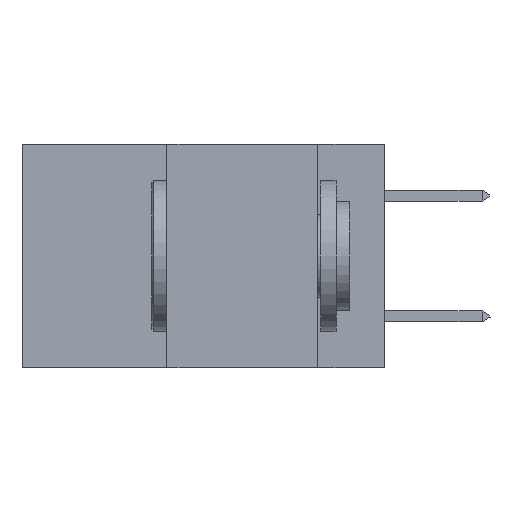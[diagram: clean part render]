
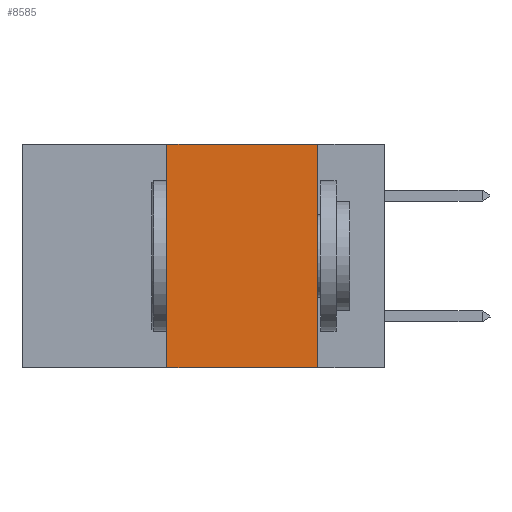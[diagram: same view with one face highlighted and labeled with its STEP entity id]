
A CAD part, left-side view. The second image highlights one B-rep face of the part: STEP entity #8585.
In plain terms, the highlighted planar face has unit normal (-1, 0, 0).
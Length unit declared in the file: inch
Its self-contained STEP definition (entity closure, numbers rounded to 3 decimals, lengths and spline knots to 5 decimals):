
#715 = EDGE_CURVE ( 'NONE', #1308, #7889, #6075, .T. ) ;
#1003 = DIRECTION ( 'NONE',  ( 0., 0., -1. ) ) ;
#1058 = EDGE_CURVE ( 'NONE', #6258, #7382, #5250, .T. ) ;
#1162 = CARTESIAN_POINT ( 'NONE',  ( 0., 0.36, 0. ) ) ;
#1308 = VERTEX_POINT ( 'NONE', #2373 ) ;
#1417 = CARTESIAN_POINT ( 'NONE',  ( 0., 0.6, 0. ) ) ;
#1742 = FACE_OUTER_BOUND ( 'NONE', #2367, .T. ) ;
#2048 = CARTESIAN_POINT ( 'NONE',  ( 0., 0.11, -0.37 ) ) ;
#2242 = LINE ( 'NONE', #1417, #4267 ) ;
#2367 = EDGE_LOOP ( 'NONE', ( #5411, #7653, #5882, #7898 ) ) ;
#2373 = CARTESIAN_POINT ( 'NONE',  ( 0., 0.11, 0. ) ) ;
#2966 = CARTESIAN_POINT ( 'NONE',  ( 0., 0.36, -0.37 ) ) ;
#4060 = VECTOR ( 'NONE', #1003, 39.37008 ) ;
#4223 = LINE ( 'NONE', #5939, #6003 ) ;
#4267 = VECTOR ( 'NONE', #5977, 39.37008 ) ;
#4809 = DIRECTION ( 'NONE',  ( 0., 0., -1. ) ) ;
#5250 = LINE ( 'NONE', #1162, #9048 ) ;
#5411 = ORIENTED_EDGE ( 'NONE', *, *, #715, .F. ) ;
#5588 = EDGE_CURVE ( 'NONE', #7382, #1308, #2242, .T. ) ;
#5747 = AXIS2_PLACEMENT_3D ( 'NONE', #6302, #9362, #4809 ) ;
#5882 = ORIENTED_EDGE ( 'NONE', *, *, #1058, .F. ) ;
#5939 = CARTESIAN_POINT ( 'NONE',  ( 0., 0.6, -0.37 ) ) ;
#5977 = DIRECTION ( 'NONE',  ( 0., -1., 0. ) ) ;
#6003 = VECTOR ( 'NONE', #6695, 39.37008 ) ;
#6075 = LINE ( 'NONE', #9231, #4060 ) ;
#6258 = VERTEX_POINT ( 'NONE', #2966 ) ;
#6302 = CARTESIAN_POINT ( 'NONE',  ( 0., 0.6, 0. ) ) ;
#6511 = DIRECTION ( 'NONE',  ( 0., 0., 1. ) ) ;
#6695 = DIRECTION ( 'NONE',  ( 0., -1., 0. ) ) ;
#7382 = VERTEX_POINT ( 'NONE', #8316 ) ;
#7653 = ORIENTED_EDGE ( 'NONE', *, *, #5588, .F. ) ;
#7889 = VERTEX_POINT ( 'NONE', #2048 ) ;
#7898 = ORIENTED_EDGE ( 'NONE', *, *, #9396, .T. ) ;
#8316 = CARTESIAN_POINT ( 'NONE',  ( 0., 0.36, 0. ) ) ;
#8585 = ADVANCED_FACE ( 'NONE', ( #1742 ), #8605, .F. ) ;
#8605 = PLANE ( 'NONE',  #5747 ) ;
#9048 = VECTOR ( 'NONE', #6511, 39.37008 ) ;
#9231 = CARTESIAN_POINT ( 'NONE',  ( 0., 0.11, 0. ) ) ;
#9362 = DIRECTION ( 'NONE',  ( 1., 0., 0. ) ) ;
#9396 = EDGE_CURVE ( 'NONE', #6258, #7889, #4223, .T. ) ;
